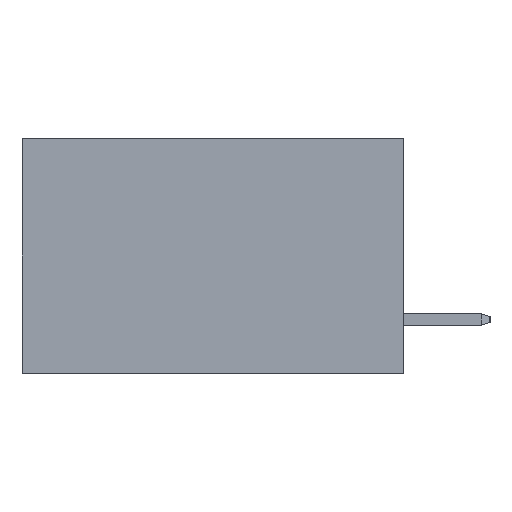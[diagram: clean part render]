
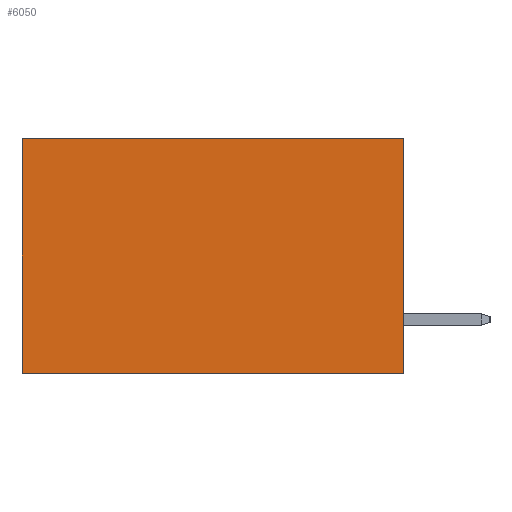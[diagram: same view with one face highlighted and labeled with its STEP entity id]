
A CAD part, left-side view. The second image highlights one B-rep face of the part: STEP entity #6050.
In plain terms, the highlighted planar face has unit normal (-1, 0, 0).
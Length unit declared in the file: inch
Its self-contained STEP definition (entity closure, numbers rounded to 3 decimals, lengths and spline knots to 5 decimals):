
#194 = DIRECTION ( 'NONE',  ( 0., 1., 0. ) ) ;
#610 = EDGE_LOOP ( 'NONE', ( #8267, #1236, #5830, #5732 ) ) ;
#1236 = ORIENTED_EDGE ( 'NONE', *, *, #1686, .F. ) ;
#1686 = EDGE_CURVE ( 'NONE', #2004, #9657, #8572, .T. ) ;
#2004 = VERTEX_POINT ( 'NONE', #3131 ) ;
#2239 = EDGE_CURVE ( 'NONE', #5357, #2004, #9466, .T. ) ;
#2607 = CARTESIAN_POINT ( 'NONE',  ( 0.2875, 0., 0. ) ) ;
#2663 = FACE_OUTER_BOUND ( 'NONE', #610, .T. ) ;
#2709 = DIRECTION ( 'NONE',  ( 0., 0., -1. ) ) ;
#2717 = LINE ( 'NONE', #5730, #4014 ) ;
#3131 = CARTESIAN_POINT ( 'NONE',  ( 0.2875, 0., -0.37 ) ) ;
#3520 = VECTOR ( 'NONE', #7783, 39.37008 ) ;
#3549 = CARTESIAN_POINT ( 'NONE',  ( 0.2875, 0., 0. ) ) ;
#3557 = DIRECTION ( 'NONE',  ( 0., 0., -1. ) ) ;
#3669 = CARTESIAN_POINT ( 'NONE',  ( 0.2875, 0.6, -0.37 ) ) ;
#4014 = VECTOR ( 'NONE', #3557, 39.37008 ) ;
#4383 = EDGE_CURVE ( 'NONE', #5447, #9657, #2717, .T. ) ;
#4792 = CARTESIAN_POINT ( 'NONE',  ( 0.2875, 0.6, 0. ) ) ;
#4811 = VECTOR ( 'NONE', #194, 39.37008 ) ;
#4929 = PLANE ( 'NONE',  #6877 ) ;
#5357 = VERTEX_POINT ( 'NONE', #7723 ) ;
#5447 = VERTEX_POINT ( 'NONE', #4792 ) ;
#5730 = CARTESIAN_POINT ( 'NONE',  ( 0.2875, 0.6, 0. ) ) ;
#5732 = ORIENTED_EDGE ( 'NONE', *, *, #5875, .T. ) ;
#5830 = ORIENTED_EDGE ( 'NONE', *, *, #2239, .F. ) ;
#5875 = EDGE_CURVE ( 'NONE', #5357, #5447, #9203, .T. ) ;
#6050 = ADVANCED_FACE ( 'NONE', ( #2663 ), #4929, .F. ) ;
#6877 = AXIS2_PLACEMENT_3D ( 'NONE', #3549, #7998, #2709 ) ;
#7474 = VECTOR ( 'NONE', #9358, 39.37008 ) ;
#7723 = CARTESIAN_POINT ( 'NONE',  ( 0.2875, 0., 0. ) ) ;
#7783 = DIRECTION ( 'NONE',  ( 0., 1., 0. ) ) ;
#7966 = CARTESIAN_POINT ( 'NONE',  ( 0.2875, 0., 0. ) ) ;
#7998 = DIRECTION ( 'NONE',  ( 1., 0., 0. ) ) ;
#8267 = ORIENTED_EDGE ( 'NONE', *, *, #4383, .T. ) ;
#8572 = LINE ( 'NONE', #8729, #3520 ) ;
#8729 = CARTESIAN_POINT ( 'NONE',  ( 0.2875, 0., -0.37 ) ) ;
#9203 = LINE ( 'NONE', #2607, #4811 ) ;
#9358 = DIRECTION ( 'NONE',  ( 0., 0., -1. ) ) ;
#9466 = LINE ( 'NONE', #7966, #7474 ) ;
#9657 = VERTEX_POINT ( 'NONE', #3669 ) ;
